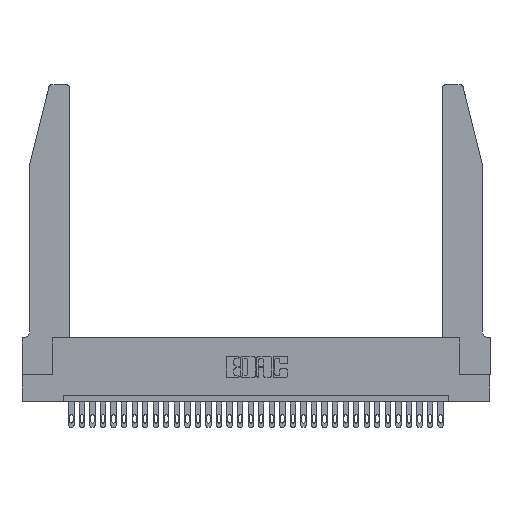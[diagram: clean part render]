
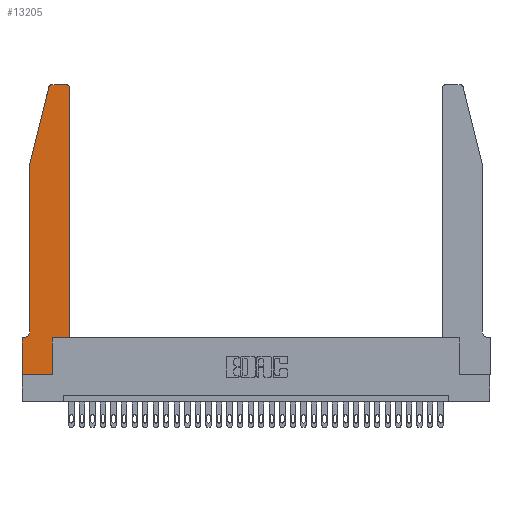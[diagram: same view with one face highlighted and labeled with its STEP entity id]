
A CAD part, top view. The second image highlights one B-rep face of the part: STEP entity #13205.
In plain terms, the highlighted planar face has unit normal (0, 0, 1).
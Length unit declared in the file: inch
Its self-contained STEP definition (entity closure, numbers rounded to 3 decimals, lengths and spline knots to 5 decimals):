
#786 = CARTESIAN_POINT ( 'NONE',  ( 0.4505, 0.35, 0.37 ) ) ;
#853 = CARTESIAN_POINT ( 'NONE',  ( 0.0755, 2., 0.37 ) ) ;
#868 = EDGE_CURVE ( 'NONE', #3837, #19046, #12148, .T. ) ;
#1203 = AXIS2_PLACEMENT_3D ( 'NONE', #10333, #17611, #2852 ) ;
#1357 = LINE ( 'NONE', #11442, #13198 ) ;
#1640 = CARTESIAN_POINT ( 'NONE',  ( 0., 0.35, 0.37 ) ) ;
#1668 = CARTESIAN_POINT ( 'NONE',  ( 0., 0.35, 0.37 ) ) ;
#1738 = VERTEX_POINT ( 'NONE', #24244 ) ;
#1818 = ORIENTED_EDGE ( 'NONE', *, *, #22991, .T. ) ;
#2208 = ORIENTED_EDGE ( 'NONE', *, *, #868, .T. ) ;
#2287 = CARTESIAN_POINT ( 'NONE',  ( 0.0755, 2., 0.37 ) ) ;
#2800 = VECTOR ( 'NONE', #20837, 39.37008 ) ;
#2852 = DIRECTION ( 'NONE',  ( 1., 0., 0. ) ) ;
#3091 = LINE ( 'NONE', #30556, #13703 ) ;
#3364 = CIRCLE ( 'NONE', #9046, 0.07 ) ;
#3837 = VERTEX_POINT ( 'NONE', #18364 ) ;
#4412 = EDGE_CURVE ( 'NONE', #11555, #3837, #21207, .T. ) ;
#4736 = VECTOR ( 'NONE', #23929, 39.37008 ) ;
#6146 = CARTESIAN_POINT ( 'NONE',  ( 0.0055, 0.42, 0.37 ) ) ;
#6570 = LINE ( 'NONE', #18942, #16014 ) ;
#7071 = ORIENTED_EDGE ( 'NONE', *, *, #17869, .T. ) ;
#7652 = LINE ( 'NONE', #32195, #22190 ) ;
#7981 = CARTESIAN_POINT ( 'NONE',  ( 0.0055, 0.35, 0.37 ) ) ;
#8011 = AXIS2_PLACEMENT_3D ( 'NONE', #1668, #13875, #14324 ) ;
#8176 = ORIENTED_EDGE ( 'NONE', *, *, #13802, .T. ) ;
#8279 = AXIS2_PLACEMENT_3D ( 'NONE', #30661, #13211, #23198 ) ;
#8308 = ORIENTED_EDGE ( 'NONE', *, *, #9580, .T. ) ;
#8952 = PLANE ( 'NONE',  #8011 ) ;
#9046 = AXIS2_PLACEMENT_3D ( 'NONE', #6146, #13727, #20893 ) ;
#9532 = ORIENTED_EDGE ( 'NONE', *, *, #4412, .T. ) ;
#9580 = EDGE_CURVE ( 'NONE', #31131, #1738, #11562, .T. ) ;
#10303 = VERTEX_POINT ( 'NONE', #22151 ) ;
#10333 = CARTESIAN_POINT ( 'NONE',  ( 0.284, 2.72, 0.37 ) ) ;
#10805 = CIRCLE ( 'NONE', #8279, 0.03 ) ;
#11221 = DIRECTION ( 'NONE',  ( 0., -1., 0. ) ) ;
#11442 = CARTESIAN_POINT ( 'NONE',  ( 0., 0., 0.37 ) ) ;
#11489 = ORIENTED_EDGE ( 'NONE', *, *, #21862, .T. ) ;
#11555 = VERTEX_POINT ( 'NONE', #13926 ) ;
#11562 = LINE ( 'NONE', #2287, #19055 ) ;
#12148 = CIRCLE ( 'NONE', #1203, 0.03 ) ;
#12200 = DIRECTION ( 'NONE',  ( 0., 1., 0. ) ) ;
#12456 = CARTESIAN_POINT ( 'NONE',  ( 0.2865, 0., 0.37 ) ) ;
#13198 = VECTOR ( 'NONE', #16958, 39.37008 ) ;
#13205 = ADVANCED_FACE ( 'NONE', ( #30553 ), #8952, .T. ) ;
#13211 = DIRECTION ( 'NONE',  ( 0., 0., 1. ) ) ;
#13703 = VECTOR ( 'NONE', #28018, 39.37008 ) ;
#13727 = DIRECTION ( 'NONE',  ( 0., 0., -1. ) ) ;
#13802 = EDGE_CURVE ( 'NONE', #27970, #14569, #18752, .T. ) ;
#13815 = EDGE_CURVE ( 'NONE', #19046, #31131, #16366, .T. ) ;
#13824 = CARTESIAN_POINT ( 'NONE',  ( 0.0755, 0.35, 0.37 ) ) ;
#13875 = DIRECTION ( 'NONE',  ( 0., 0., 1. ) ) ;
#13926 = CARTESIAN_POINT ( 'NONE',  ( 0.4205, 2.75, 0.37 ) ) ;
#14051 = CARTESIAN_POINT ( 'NONE',  ( 0., 0., 0.37 ) ) ;
#14324 = DIRECTION ( 'NONE',  ( 1., 0., 0. ) ) ;
#14369 = ORIENTED_EDGE ( 'NONE', *, *, #13815, .T. ) ;
#14385 = ORIENTED_EDGE ( 'NONE', *, *, #28435, .T. ) ;
#14569 = VERTEX_POINT ( 'NONE', #1640 ) ;
#14868 = ORIENTED_EDGE ( 'NONE', *, *, #28055, .T. ) ;
#15396 = LINE ( 'NONE', #30702, #2800 ) ;
#16014 = VECTOR ( 'NONE', #11221, 39.37008 ) ;
#16366 = LINE ( 'NONE', #853, #25775 ) ;
#16958 = DIRECTION ( 'NONE',  ( 1., 0., 0. ) ) ;
#17611 = DIRECTION ( 'NONE',  ( 0., 0., 1. ) ) ;
#17869 = EDGE_CURVE ( 'NONE', #22043, #24223, #1357, .T. ) ;
#18364 = CARTESIAN_POINT ( 'NONE',  ( 0.284, 2.75, 0.37 ) ) ;
#18752 = LINE ( 'NONE', #13824, #31292 ) ;
#18942 = CARTESIAN_POINT ( 'NONE',  ( 0., 0., 0.37 ) ) ;
#19046 = VERTEX_POINT ( 'NONE', #22725 ) ;
#19055 = VECTOR ( 'NONE', #27535, 39.37008 ) ;
#20837 = DIRECTION ( 'NONE',  ( 0., 1., 0. ) ) ;
#20893 = DIRECTION ( 'NONE',  ( -1., 0., 0. ) ) ;
#20980 = DIRECTION ( 'NONE',  ( -1., 0., 0. ) ) ;
#21207 = LINE ( 'NONE', #26346, #4736 ) ;
#21862 = EDGE_CURVE ( 'NONE', #10303, #30444, #3091, .T. ) ;
#22043 = VERTEX_POINT ( 'NONE', #14051 ) ;
#22142 = ORIENTED_EDGE ( 'NONE', *, *, #22300, .T. ) ;
#22151 = CARTESIAN_POINT ( 'NONE',  ( 0.2865, 0.35, 0.37 ) ) ;
#22190 = VECTOR ( 'NONE', #12200, 39.37008 ) ;
#22300 = EDGE_CURVE ( 'NONE', #14569, #22043, #6570, .T. ) ;
#22725 = CARTESIAN_POINT ( 'NONE',  ( 0.25487, 2.72718, 0.37 ) ) ;
#22991 = EDGE_CURVE ( 'NONE', #1738, #27970, #3364, .T. ) ;
#23198 = DIRECTION ( 'NONE',  ( 1., 0., 0. ) ) ;
#23929 = DIRECTION ( 'NONE',  ( -1., 0., 0. ) ) ;
#24223 = VERTEX_POINT ( 'NONE', #12456 ) ;
#24244 = CARTESIAN_POINT ( 'NONE',  ( 0.0755, 0.42, 0.37 ) ) ;
#25775 = VECTOR ( 'NONE', #28420, 39.37008 ) ;
#25894 = CARTESIAN_POINT ( 'NONE',  ( 0.0755, 2., 0.37 ) ) ;
#26002 = CARTESIAN_POINT ( 'NONE',  ( 0.4505, 2.72, 0.37 ) ) ;
#26346 = CARTESIAN_POINT ( 'NONE',  ( 0.2605, 2.75, 0.37 ) ) ;
#27535 = DIRECTION ( 'NONE',  ( 0., -1., 0. ) ) ;
#27970 = VERTEX_POINT ( 'NONE', #7981 ) ;
#28018 = DIRECTION ( 'NONE',  ( 1., 0., 0. ) ) ;
#28055 = EDGE_CURVE ( 'NONE', #32207, #11555, #10805, .T. ) ;
#28420 = DIRECTION ( 'NONE',  ( -0.239, -0.971, 0. ) ) ;
#28435 = EDGE_CURVE ( 'NONE', #30444, #32207, #7652, .T. ) ;
#29942 = EDGE_CURVE ( 'NONE', #24223, #10303, #15396, .T. ) ;
#30444 = VERTEX_POINT ( 'NONE', #786 ) ;
#30553 = FACE_OUTER_BOUND ( 'NONE', #31563, .T. ) ;
#30556 = CARTESIAN_POINT ( 'NONE',  ( 0.4505, 0.35, 0.37 ) ) ;
#30661 = CARTESIAN_POINT ( 'NONE',  ( 0.4205, 2.72, 0.37 ) ) ;
#30702 = CARTESIAN_POINT ( 'NONE',  ( 0.2865, 0.35, 0.37 ) ) ;
#30897 = ORIENTED_EDGE ( 'NONE', *, *, #29942, .T. ) ;
#31131 = VERTEX_POINT ( 'NONE', #25894 ) ;
#31292 = VECTOR ( 'NONE', #20980, 39.37008 ) ;
#31563 = EDGE_LOOP ( 'NONE', ( #9532, #2208, #14369, #8308, #1818, #8176, #22142, #7071, #30897, #11489, #14385, #14868 ) ) ;
#32195 = CARTESIAN_POINT ( 'NONE',  ( 0.4505, 0.35, 0.37 ) ) ;
#32207 = VERTEX_POINT ( 'NONE', #26002 ) ;
